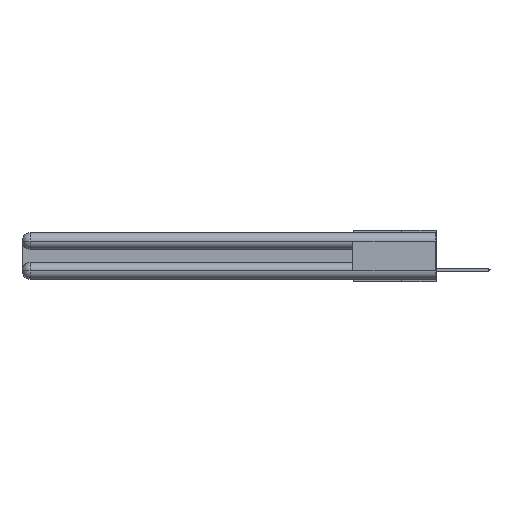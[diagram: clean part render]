
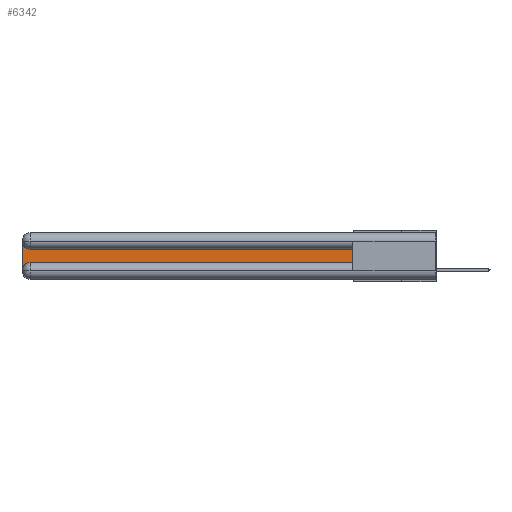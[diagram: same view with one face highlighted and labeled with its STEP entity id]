
A CAD part, left-side view. The second image highlights one B-rep face of the part: STEP entity #6342.
In plain terms, the highlighted planar face has unit normal (-1, 0, 0).
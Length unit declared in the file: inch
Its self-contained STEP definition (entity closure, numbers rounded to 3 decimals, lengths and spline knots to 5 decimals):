
#1066 = DIRECTION ( 'NONE',  ( 0., 0., -1. ) ) ;
#1218 = DIRECTION ( 'NONE',  ( 1., 0., 0. ) ) ;
#1250 = FACE_OUTER_BOUND ( 'NONE', #21850, .T. ) ;
#2047 = CARTESIAN_POINT ( 'NONE',  ( 0.075, 3., -0.1225 ) ) ;
#5851 = EDGE_CURVE ( 'NONE', #20808, #19963, #7073, .T. ) ;
#6257 = LINE ( 'NONE', #18395, #12075 ) ;
#6342 = ADVANCED_FACE ( 'NONE', ( #1250 ), #21775, .F. ) ;
#6378 = VERTEX_POINT ( 'NONE', #22633 ) ;
#6423 = DIRECTION ( 'NONE',  ( 0., 0., -1. ) ) ;
#6737 = EDGE_CURVE ( 'NONE', #6378, #20808, #13210, .T. ) ;
#7073 = CIRCLE ( 'NONE', #19127, 0.06 ) ;
#8347 = ORIENTED_EDGE ( 'NONE', *, *, #26974, .T. ) ;
#8368 = DIRECTION ( 'NONE',  ( 0., 0., 1. ) ) ;
#9110 = CARTESIAN_POINT ( 'NONE',  ( 0.075, 0.6, -0.2175 ) ) ;
#9779 = DIRECTION ( 'NONE',  ( 0., 0., -1. ) ) ;
#9979 = CIRCLE ( 'NONE', #10646, 0.06 ) ;
#10646 = AXIS2_PLACEMENT_3D ( 'NONE', #14174, #22913, #1066 ) ;
#11089 = VERTEX_POINT ( 'NONE', #9110 ) ;
#11113 = VECTOR ( 'NONE', #8368, 39.37008 ) ;
#11950 = DIRECTION ( 'NONE',  ( 0., -1., 0. ) ) ;
#12075 = VECTOR ( 'NONE', #11950, 39.37008 ) ;
#13210 = LINE ( 'NONE', #13411, #28309 ) ;
#13411 = CARTESIAN_POINT ( 'NONE',  ( 0.075, 3., -0.2175 ) ) ;
#13646 = AXIS2_PLACEMENT_3D ( 'NONE', #2047, #14852, #17363 ) ;
#14174 = CARTESIAN_POINT ( 'NONE',  ( 0.075, 2.94, -0.0625 ) ) ;
#14310 = CARTESIAN_POINT ( 'NONE',  ( 0.075, 2.94, -0.2775 ) ) ;
#14852 = DIRECTION ( 'NONE',  ( 1., 0., 0. ) ) ;
#15584 = EDGE_CURVE ( 'NONE', #11089, #18870, #18345, .T. ) ;
#16140 = CARTESIAN_POINT ( 'NONE',  ( 0.075, 2.94, -0.2175 ) ) ;
#16262 = ORIENTED_EDGE ( 'NONE', *, *, #6737, .T. ) ;
#16603 = CARTESIAN_POINT ( 'NONE',  ( 0.075, 3., -0.2775 ) ) ;
#16871 = EDGE_CURVE ( 'NONE', #18870, #22019, #24123, .T. ) ;
#17274 = ORIENTED_EDGE ( 'NONE', *, *, #15584, .T. ) ;
#17363 = DIRECTION ( 'NONE',  ( 0., 0., -1. ) ) ;
#17876 = EDGE_CURVE ( 'NONE', #22019, #6378, #9979, .T. ) ;
#18345 = LINE ( 'NONE', #27745, #11113 ) ;
#18395 = CARTESIAN_POINT ( 'NONE',  ( 0.075, 0.6, -0.2175 ) ) ;
#18870 = VERTEX_POINT ( 'NONE', #23888 ) ;
#18884 = CARTESIAN_POINT ( 'NONE',  ( 0.075, 2.94, -0.1225 ) ) ;
#19127 = AXIS2_PLACEMENT_3D ( 'NONE', #14310, #1218, #9779 ) ;
#19963 = VERTEX_POINT ( 'NONE', #16140 ) ;
#20173 = ORIENTED_EDGE ( 'NONE', *, *, #17876, .T. ) ;
#20808 = VERTEX_POINT ( 'NONE', #16603 ) ;
#21444 = ORIENTED_EDGE ( 'NONE', *, *, #16871, .T. ) ;
#21478 = DIRECTION ( 'NONE',  ( 0., 1., 0. ) ) ;
#21775 = PLANE ( 'NONE',  #13646 ) ;
#21850 = EDGE_LOOP ( 'NONE', ( #21444, #20173, #16262, #24183, #8347, #17274 ) ) ;
#22019 = VERTEX_POINT ( 'NONE', #18884 ) ;
#22633 = CARTESIAN_POINT ( 'NONE',  ( 0.075, 3., -0.0625 ) ) ;
#22913 = DIRECTION ( 'NONE',  ( 1., 0., 0. ) ) ;
#23526 = CARTESIAN_POINT ( 'NONE',  ( 0.075, 0.6, -0.1225 ) ) ;
#23888 = CARTESIAN_POINT ( 'NONE',  ( 0.075, 0.6, -0.1225 ) ) ;
#24123 = LINE ( 'NONE', #23526, #26197 ) ;
#24183 = ORIENTED_EDGE ( 'NONE', *, *, #5851, .T. ) ;
#26197 = VECTOR ( 'NONE', #21478, 39.37008 ) ;
#26974 = EDGE_CURVE ( 'NONE', #19963, #11089, #6257, .T. ) ;
#27745 = CARTESIAN_POINT ( 'NONE',  ( 0.075, 0.6, -0.2175 ) ) ;
#28309 = VECTOR ( 'NONE', #6423, 39.37008 ) ;
